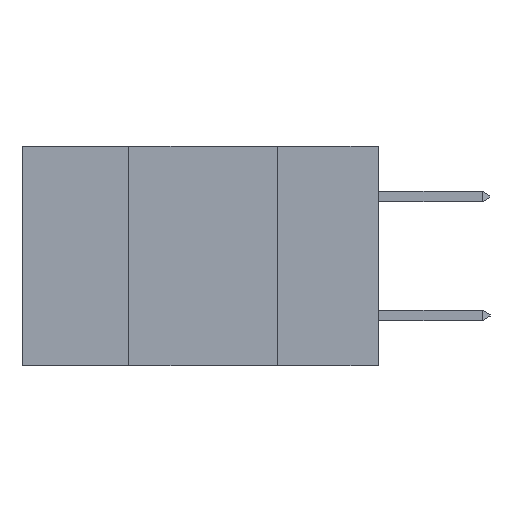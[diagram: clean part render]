
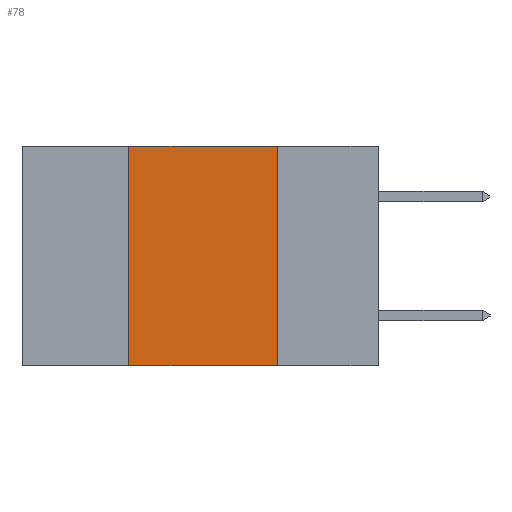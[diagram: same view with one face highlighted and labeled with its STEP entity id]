
A CAD part, left-side view. The second image highlights one B-rep face of the part: STEP entity #78.
In plain terms, the highlighted planar face has unit normal (-1, 0, 0).
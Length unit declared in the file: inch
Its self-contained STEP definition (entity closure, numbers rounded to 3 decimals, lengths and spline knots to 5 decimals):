
#71 = EDGE_CURVE ( 'NONE', #5985, #2382, #1227, .T. ) ;
#78 = ADVANCED_FACE ( 'NONE', ( #13689 ), #5575, .F. ) ;
#735 = DIRECTION ( 'NONE',  ( 0., 0., -1. ) ) ;
#868 = DIRECTION ( 'NONE',  ( 0., 0., -1. ) ) ;
#873 = CARTESIAN_POINT ( 'NONE',  ( 0., 0.17, 0. ) ) ;
#1227 = LINE ( 'NONE', #4222, #13353 ) ;
#1542 = ORIENTED_EDGE ( 'NONE', *, *, #71, .F. ) ;
#1599 = VECTOR ( 'NONE', #4853, 39.37008 ) ;
#1644 = ORIENTED_EDGE ( 'NONE', *, *, #9121, .F. ) ;
#1961 = LINE ( 'NONE', #8479, #1599 ) ;
#2034 = DIRECTION ( 'NONE',  ( 1., 0., 0. ) ) ;
#2169 = ORIENTED_EDGE ( 'NONE', *, *, #6760, .F. ) ;
#2218 = CARTESIAN_POINT ( 'NONE',  ( 0., 0.6, 0. ) ) ;
#2382 = VERTEX_POINT ( 'NONE', #10134 ) ;
#2487 = LINE ( 'NONE', #14183, #8889 ) ;
#2942 = ORIENTED_EDGE ( 'NONE', *, *, #14000, .T. ) ;
#3203 = EDGE_LOOP ( 'NONE', ( #1542, #1644, #2169, #2942 ) ) ;
#3525 = DIRECTION ( 'NONE',  ( 0., 0., 1. ) ) ;
#4098 = CARTESIAN_POINT ( 'NONE',  ( 0., 0.42, -0.37 ) ) ;
#4222 = CARTESIAN_POINT ( 'NONE',  ( 0., 0.17, -0.37 ) ) ;
#4853 = DIRECTION ( 'NONE',  ( 0., -1., 0. ) ) ;
#5575 = PLANE ( 'NONE',  #11815 ) ;
#5985 = VERTEX_POINT ( 'NONE', #873 ) ;
#6328 = LINE ( 'NONE', #4098, #12186 ) ;
#6760 = EDGE_CURVE ( 'NONE', #15094, #9421, #6328, .T. ) ;
#8479 = CARTESIAN_POINT ( 'NONE',  ( 0., 0.6, -0.37 ) ) ;
#8889 = VECTOR ( 'NONE', #14277, 39.37008 ) ;
#9121 = EDGE_CURVE ( 'NONE', #9421, #5985, #2487, .T. ) ;
#9421 = VERTEX_POINT ( 'NONE', #12190 ) ;
#10134 = CARTESIAN_POINT ( 'NONE',  ( 0., 0.17, -0.37 ) ) ;
#11815 = AXIS2_PLACEMENT_3D ( 'NONE', #2218, #2034, #735 ) ;
#12057 = CARTESIAN_POINT ( 'NONE',  ( 0., 0.42, -0.37 ) ) ;
#12186 = VECTOR ( 'NONE', #3525, 39.37008 ) ;
#12190 = CARTESIAN_POINT ( 'NONE',  ( 0., 0.42, 0. ) ) ;
#13353 = VECTOR ( 'NONE', #868, 39.37008 ) ;
#13689 = FACE_OUTER_BOUND ( 'NONE', #3203, .T. ) ;
#14000 = EDGE_CURVE ( 'NONE', #15094, #2382, #1961, .T. ) ;
#14183 = CARTESIAN_POINT ( 'NONE',  ( 0., 0.6, 0. ) ) ;
#14277 = DIRECTION ( 'NONE',  ( 0., -1., 0. ) ) ;
#15094 = VERTEX_POINT ( 'NONE', #12057 ) ;
